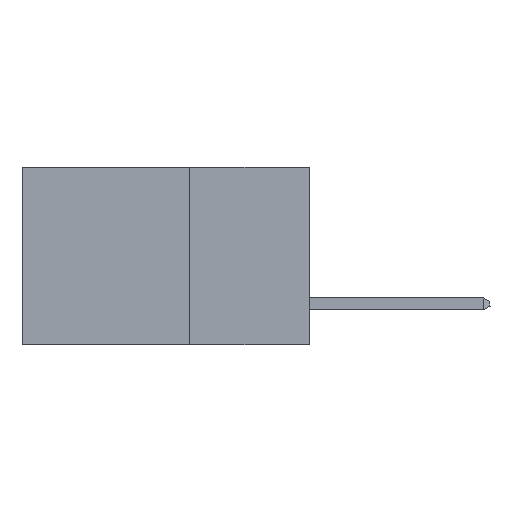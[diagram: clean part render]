
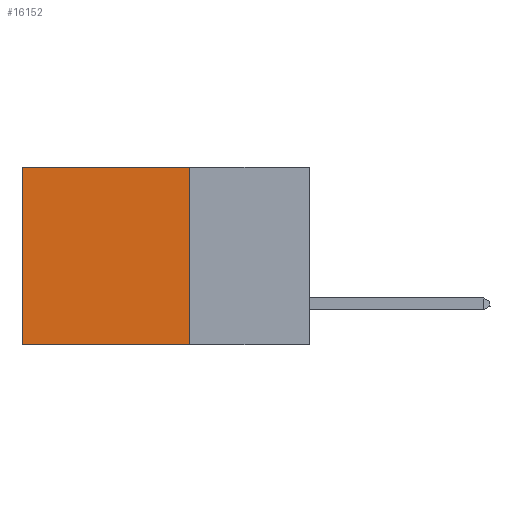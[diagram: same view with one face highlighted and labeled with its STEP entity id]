
A CAD part, left-side view. The second image highlights one B-rep face of the part: STEP entity #16152.
In plain terms, the highlighted planar face has unit normal (-1, 0, 0).
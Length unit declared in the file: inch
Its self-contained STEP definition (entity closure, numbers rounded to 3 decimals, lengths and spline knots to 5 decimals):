
#320 = EDGE_CURVE ( 'NONE', #19624, #1454, #9025, .T. ) ;
#453 = LINE ( 'NONE', #5922, #14013 ) ;
#1454 = VERTEX_POINT ( 'NONE', #16324 ) ;
#2325 = ORIENTED_EDGE ( 'NONE', *, *, #10675, .T. ) ;
#2383 = VECTOR ( 'NONE', #8584, 39.37008 ) ;
#3584 = CARTESIAN_POINT ( 'NONE',  ( 0.2875, 0.25, 0. ) ) ;
#3951 = LINE ( 'NONE', #15924, #15282 ) ;
#5372 = EDGE_CURVE ( 'NONE', #19624, #18181, #3951, .T. ) ;
#5922 = CARTESIAN_POINT ( 'NONE',  ( 0.2875, 0.25, -0.37 ) ) ;
#6242 = CARTESIAN_POINT ( 'NONE',  ( 0.2875, 0.25, 0. ) ) ;
#6591 = FACE_OUTER_BOUND ( 'NONE', #10236, .T. ) ;
#6832 = ORIENTED_EDGE ( 'NONE', *, *, #17195, .F. ) ;
#8063 = DIRECTION ( 'NONE',  ( 1., 0., 0. ) ) ;
#8584 = DIRECTION ( 'NONE',  ( 0., 0., -1. ) ) ;
#9025 = LINE ( 'NONE', #14480, #22628 ) ;
#10236 = EDGE_LOOP ( 'NONE', ( #2325, #6832, #10359, #18238 ) ) ;
#10359 = ORIENTED_EDGE ( 'NONE', *, *, #320, .F. ) ;
#10675 = EDGE_CURVE ( 'NONE', #18181, #10924, #12094, .T. ) ;
#10924 = VERTEX_POINT ( 'NONE', #21404 ) ;
#12094 = LINE ( 'NONE', #20865, #2383 ) ;
#12809 = CARTESIAN_POINT ( 'NONE',  ( 0.2875, 0.6, 0. ) ) ;
#14013 = VECTOR ( 'NONE', #22089, 39.37008 ) ;
#14480 = CARTESIAN_POINT ( 'NONE',  ( 0.2875, 0.25, 0. ) ) ;
#15052 = AXIS2_PLACEMENT_3D ( 'NONE', #6242, #8063, #20568 ) ;
#15282 = VECTOR ( 'NONE', #19504, 39.37008 ) ;
#15924 = CARTESIAN_POINT ( 'NONE',  ( 0.2875, 0.25, 0. ) ) ;
#16152 = ADVANCED_FACE ( 'NONE', ( #6591 ), #16794, .F. ) ;
#16324 = CARTESIAN_POINT ( 'NONE',  ( 0.2875, 0.25, -0.37 ) ) ;
#16794 = PLANE ( 'NONE',  #15052 ) ;
#17195 = EDGE_CURVE ( 'NONE', #1454, #10924, #453, .T. ) ;
#18181 = VERTEX_POINT ( 'NONE', #12809 ) ;
#18238 = ORIENTED_EDGE ( 'NONE', *, *, #5372, .T. ) ;
#19504 = DIRECTION ( 'NONE',  ( 0., 1., 0. ) ) ;
#19624 = VERTEX_POINT ( 'NONE', #3584 ) ;
#20568 = DIRECTION ( 'NONE',  ( 0., 0., -1. ) ) ;
#20865 = CARTESIAN_POINT ( 'NONE',  ( 0.2875, 0.6, 0. ) ) ;
#21404 = CARTESIAN_POINT ( 'NONE',  ( 0.2875, 0.6, -0.37 ) ) ;
#22089 = DIRECTION ( 'NONE',  ( 0., 1., 0. ) ) ;
#22520 = DIRECTION ( 'NONE',  ( 0., 0., -1. ) ) ;
#22628 = VECTOR ( 'NONE', #22520, 39.37008 ) ;
